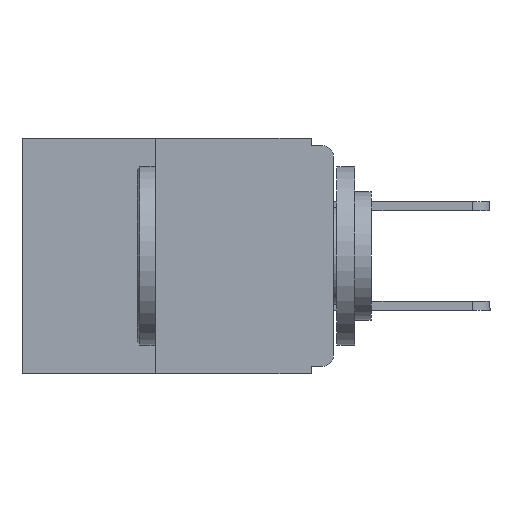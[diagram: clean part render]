
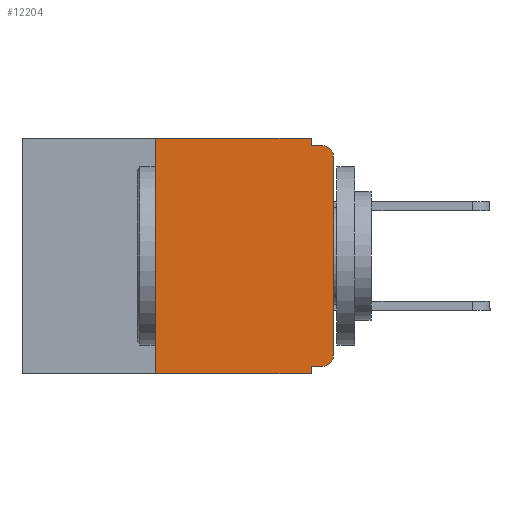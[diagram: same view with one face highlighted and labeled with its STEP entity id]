
A CAD part, left-side view. The second image highlights one B-rep face of the part: STEP entity #12204.
In plain terms, the highlighted planar face has unit normal (-1, 0, 0).
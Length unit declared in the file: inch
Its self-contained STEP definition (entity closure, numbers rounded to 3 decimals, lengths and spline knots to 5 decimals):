
#55 = ORIENTED_EDGE ( 'NONE', *, *, #16158, .T. ) ;
#124 = EDGE_CURVE ( 'NONE', #13876, #14600, #1648, .T. ) ;
#168 = CARTESIAN_POINT ( 'NONE',  ( 0., 0., 0. ) ) ;
#213 = CARTESIAN_POINT ( 'NONE',  ( 0., 0.015, -0.01 ) ) ;
#216 = VERTEX_POINT ( 'NONE', #7702 ) ;
#342 = CARTESIAN_POINT ( 'NONE',  ( 0., 0.25, -0.33 ) ) ;
#420 = CARTESIAN_POINT ( 'NONE',  ( 0., 0.25, -0.33 ) ) ;
#797 = CARTESIAN_POINT ( 'NONE',  ( 0., 0.031, -0.33 ) ) ;
#1244 = CARTESIAN_POINT ( 'NONE',  ( 0., 0.031, 0. ) ) ;
#1361 = LINE ( 'NONE', #6706, #11323 ) ;
#1634 = VECTOR ( 'NONE', #6298, 39.37008 ) ;
#1648 = LINE ( 'NONE', #15013, #4843 ) ;
#1697 = DIRECTION ( 'NONE',  ( 0., 0., 1. ) ) ;
#2324 = VERTEX_POINT ( 'NONE', #1244 ) ;
#2353 = CARTESIAN_POINT ( 'NONE',  ( 0., 0.015, -0.305 ) ) ;
#2703 = VECTOR ( 'NONE', #4275, 39.37008 ) ;
#2997 = ORIENTED_EDGE ( 'NONE', *, *, #5021, .F. ) ;
#3068 = LINE ( 'NONE', #342, #6290 ) ;
#3231 = AXIS2_PLACEMENT_3D ( 'NONE', #15547, #16891, #8878 ) ;
#3335 = EDGE_CURVE ( 'NONE', #5612, #4641, #8415, .T. ) ;
#3444 = ORIENTED_EDGE ( 'NONE', *, *, #9872, .T. ) ;
#3742 = DIRECTION ( 'NONE',  ( 0., 0., -1. ) ) ;
#4275 = DIRECTION ( 'NONE',  ( 0., 0., 1. ) ) ;
#4641 = VERTEX_POINT ( 'NONE', #797 ) ;
#4717 = CARTESIAN_POINT ( 'NONE',  ( 0., 0.015, -0.025 ) ) ;
#4843 = VECTOR ( 'NONE', #11734, 39.37008 ) ;
#4856 = CARTESIAN_POINT ( 'NONE',  ( 0., 0., -0.025 ) ) ;
#4949 = ORIENTED_EDGE ( 'NONE', *, *, #16510, .F. ) ;
#5021 = EDGE_CURVE ( 'NONE', #8897, #17452, #10471, .T. ) ;
#5612 = VERTEX_POINT ( 'NONE', #420 ) ;
#5665 = DIRECTION ( 'NONE',  ( 0., 0., -1. ) ) ;
#5770 = VECTOR ( 'NONE', #5665, 39.37008 ) ;
#5777 = ORIENTED_EDGE ( 'NONE', *, *, #3335, .T. ) ;
#6071 = DIRECTION ( 'NONE',  ( 0., 0., -1. ) ) ;
#6155 = PLANE ( 'NONE',  #3231 ) ;
#6290 = VECTOR ( 'NONE', #1697, 39.37008 ) ;
#6298 = DIRECTION ( 'NONE',  ( 0., -1., 0. ) ) ;
#6342 = LINE ( 'NONE', #168, #2703 ) ;
#6675 = DIRECTION ( 'NONE',  ( 0., 1., 0. ) ) ;
#6706 = CARTESIAN_POINT ( 'NONE',  ( 0., 0.031, 0. ) ) ;
#6829 = EDGE_CURVE ( 'NONE', #17452, #4641, #9368, .T. ) ;
#7484 = CARTESIAN_POINT ( 'NONE',  ( 0., 0.031, -0.32 ) ) ;
#7702 = CARTESIAN_POINT ( 'NONE',  ( 0., 0., -0.305 ) ) ;
#7910 = EDGE_LOOP ( 'NONE', ( #13592, #55, #11731, #4949, #8963, #16082, #5777, #13404, #2997, #3444 ) ) ;
#7971 = EDGE_CURVE ( 'NONE', #10346, #2324, #8264, .T. ) ;
#8264 = LINE ( 'NONE', #12338, #14984 ) ;
#8415 = LINE ( 'NONE', #12773, #1634 ) ;
#8797 = CARTESIAN_POINT ( 'NONE',  ( 0., 0., -0.32 ) ) ;
#8878 = DIRECTION ( 'NONE',  ( 0., 0., -1. ) ) ;
#8897 = VERTEX_POINT ( 'NONE', #12845 ) ;
#8963 = ORIENTED_EDGE ( 'NONE', *, *, #7971, .F. ) ;
#9368 = LINE ( 'NONE', #11034, #5770 ) ;
#9469 = AXIS2_PLACEMENT_3D ( 'NONE', #4717, #14138, #6071 ) ;
#9872 = EDGE_CURVE ( 'NONE', #8897, #216, #10650, .T. ) ;
#10346 = VERTEX_POINT ( 'NONE', #14461 ) ;
#10471 = LINE ( 'NONE', #8797, #13632 ) ;
#10490 = CIRCLE ( 'NONE', #9469, 0.015 ) ;
#10650 = CIRCLE ( 'NONE', #17095, 0.015 ) ;
#11034 = CARTESIAN_POINT ( 'NONE',  ( 0., 0.031, -0.33 ) ) ;
#11323 = VECTOR ( 'NONE', #17444, 39.37008 ) ;
#11731 = ORIENTED_EDGE ( 'NONE', *, *, #124, .F. ) ;
#11734 = DIRECTION ( 'NONE',  ( 0., -1., 0. ) ) ;
#11876 = DIRECTION ( 'NONE',  ( -1., 0., 0. ) ) ;
#11953 = EDGE_CURVE ( 'NONE', #216, #12217, #6342, .T. ) ;
#12204 = ADVANCED_FACE ( 'NONE', ( #12911 ), #6155, .F. ) ;
#12217 = VERTEX_POINT ( 'NONE', #4856 ) ;
#12231 = CARTESIAN_POINT ( 'NONE',  ( 0., 0.031, -0.01 ) ) ;
#12338 = CARTESIAN_POINT ( 'NONE',  ( 0., 0.437, 0. ) ) ;
#12773 = CARTESIAN_POINT ( 'NONE',  ( 0., 0.437, -0.33 ) ) ;
#12845 = CARTESIAN_POINT ( 'NONE',  ( 0., 0.015, -0.32 ) ) ;
#12911 = FACE_OUTER_BOUND ( 'NONE', #7910, .T. ) ;
#13404 = ORIENTED_EDGE ( 'NONE', *, *, #6829, .F. ) ;
#13592 = ORIENTED_EDGE ( 'NONE', *, *, #11953, .T. ) ;
#13632 = VECTOR ( 'NONE', #6675, 39.37008 ) ;
#13663 = DIRECTION ( 'NONE',  ( 0., -1., 0. ) ) ;
#13876 = VERTEX_POINT ( 'NONE', #12231 ) ;
#14138 = DIRECTION ( 'NONE',  ( -1., 0., 0. ) ) ;
#14461 = CARTESIAN_POINT ( 'NONE',  ( 0., 0.25, 0. ) ) ;
#14600 = VERTEX_POINT ( 'NONE', #213 ) ;
#14984 = VECTOR ( 'NONE', #13663, 39.37008 ) ;
#15013 = CARTESIAN_POINT ( 'NONE',  ( 0., 0., -0.01 ) ) ;
#15511 = EDGE_CURVE ( 'NONE', #5612, #10346, #3068, .T. ) ;
#15547 = CARTESIAN_POINT ( 'NONE',  ( 0., 0.437, 0. ) ) ;
#16082 = ORIENTED_EDGE ( 'NONE', *, *, #15511, .F. ) ;
#16158 = EDGE_CURVE ( 'NONE', #12217, #14600, #10490, .T. ) ;
#16510 = EDGE_CURVE ( 'NONE', #2324, #13876, #1361, .T. ) ;
#16891 = DIRECTION ( 'NONE',  ( 1., 0., 0. ) ) ;
#17095 = AXIS2_PLACEMENT_3D ( 'NONE', #2353, #11876, #3742 ) ;
#17444 = DIRECTION ( 'NONE',  ( 0., 0., -1. ) ) ;
#17452 = VERTEX_POINT ( 'NONE', #7484 ) ;
